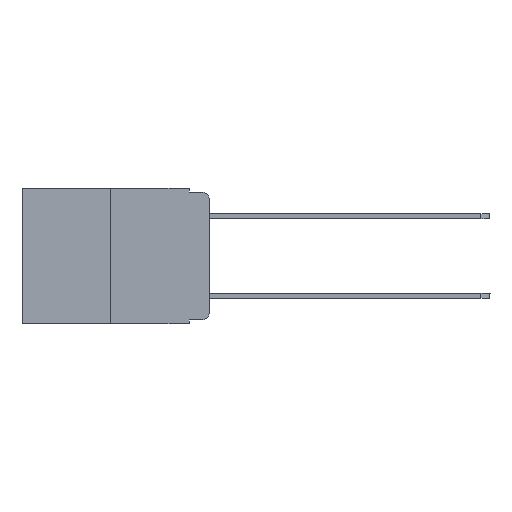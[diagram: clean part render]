
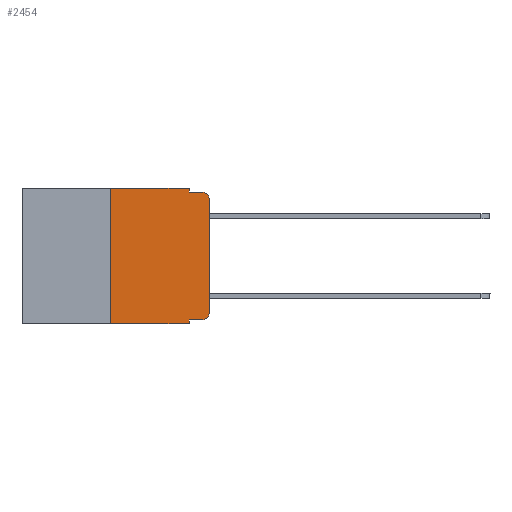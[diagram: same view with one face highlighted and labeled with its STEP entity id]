
A CAD part, left-side view. The second image highlights one B-rep face of the part: STEP entity #2454.
In plain terms, the highlighted planar face has unit normal (-1, 0, 0).
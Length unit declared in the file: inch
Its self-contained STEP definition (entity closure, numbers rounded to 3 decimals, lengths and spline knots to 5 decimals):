
#126 = VERTEX_POINT ( 'NONE', #4858 ) ;
#336 = ORIENTED_EDGE ( 'NONE', *, *, #6059, .T. ) ;
#388 = ORIENTED_EDGE ( 'NONE', *, *, #6709, .T. ) ;
#465 = EDGE_LOOP ( 'NONE', ( #6088, #12707, #9747, #11387, #4424, #7890, #388, #7771, #10635, #336 ) ) ;
#998 = CARTESIAN_POINT ( 'NONE',  ( 0., 0.02, -0.313 ) ) ;
#1402 = CARTESIAN_POINT ( 'NONE',  ( 0., 0.02, -0.01 ) ) ;
#1640 = EDGE_CURVE ( 'NONE', #2053, #11706, #2473, .T. ) ;
#1708 = AXIS2_PLACEMENT_3D ( 'NONE', #2082, #2881, #10051 ) ;
#1828 = CARTESIAN_POINT ( 'NONE',  ( 0., 0., 0. ) ) ;
#2053 = VERTEX_POINT ( 'NONE', #12426 ) ;
#2082 = CARTESIAN_POINT ( 'NONE',  ( 0., 0.473, 0. ) ) ;
#2126 = LINE ( 'NONE', #8281, #8659 ) ;
#2194 = DIRECTION ( 'NONE',  ( 0., 0., -1. ) ) ;
#2251 = DIRECTION ( 'NONE',  ( 0., -1., 0. ) ) ;
#2450 = CARTESIAN_POINT ( 'NONE',  ( 0., 0.02, -0.333 ) ) ;
#2454 = ADVANCED_FACE ( 'NONE', ( #8114 ), #12247, .F. ) ;
#2473 = CIRCLE ( 'NONE', #4181, 0.02 ) ;
#2568 = VERTEX_POINT ( 'NONE', #12329 ) ;
#2829 = EDGE_CURVE ( 'NONE', #126, #2053, #10996, .T. ) ;
#2830 = LINE ( 'NONE', #11875, #12501 ) ;
#2881 = DIRECTION ( 'NONE',  ( 1., 0., 0. ) ) ;
#2900 = DIRECTION ( 'NONE',  ( 0., -1., 0. ) ) ;
#3019 = EDGE_CURVE ( 'NONE', #10399, #3086, #12302, .T. ) ;
#3086 = VERTEX_POINT ( 'NONE', #3205 ) ;
#3125 = VECTOR ( 'NONE', #7096, 39.37008 ) ;
#3205 = CARTESIAN_POINT ( 'NONE',  ( 0., 0.25, 0. ) ) ;
#3327 = DIRECTION ( 'NONE',  ( -1., 0., 0. ) ) ;
#3738 = CARTESIAN_POINT ( 'NONE',  ( 0., 0.051, 0. ) ) ;
#3748 = CARTESIAN_POINT ( 'NONE',  ( 0., 0.051, 0. ) ) ;
#3861 = VERTEX_POINT ( 'NONE', #10927 ) ;
#3913 = VECTOR ( 'NONE', #8777, 39.37008 ) ;
#4181 = AXIS2_PLACEMENT_3D ( 'NONE', #9445, #3327, #2194 ) ;
#4343 = VERTEX_POINT ( 'NONE', #3748 ) ;
#4424 = ORIENTED_EDGE ( 'NONE', *, *, #11277, .F. ) ;
#4569 = CARTESIAN_POINT ( 'NONE',  ( 0., 0.051, -0.343 ) ) ;
#4829 = LINE ( 'NONE', #12912, #8222 ) ;
#4858 = CARTESIAN_POINT ( 'NONE',  ( 0., 0., -0.313 ) ) ;
#5090 = DIRECTION ( 'NONE',  ( -1., 0., 0. ) ) ;
#5369 = VERTEX_POINT ( 'NONE', #4569 ) ;
#5817 = EDGE_CURVE ( 'NONE', #4343, #2568, #9903, .T. ) ;
#5929 = EDGE_CURVE ( 'NONE', #3861, #5369, #9705, .T. ) ;
#6059 = EDGE_CURVE ( 'NONE', #7695, #126, #11404, .T. ) ;
#6088 = ORIENTED_EDGE ( 'NONE', *, *, #2829, .T. ) ;
#6276 = CARTESIAN_POINT ( 'NONE',  ( 0., 0.473, 0. ) ) ;
#6494 = CARTESIAN_POINT ( 'NONE',  ( 0., 0.25, -0.343 ) ) ;
#6709 = EDGE_CURVE ( 'NONE', #10399, #5369, #4829, .T. ) ;
#6982 = VECTOR ( 'NONE', #2251, 39.37008 ) ;
#7096 = DIRECTION ( 'NONE',  ( 0., 0., 1. ) ) ;
#7585 = EDGE_CURVE ( 'NONE', #2568, #11706, #2126, .T. ) ;
#7695 = VERTEX_POINT ( 'NONE', #2450 ) ;
#7738 = DIRECTION ( 'NONE',  ( 0., -1., 0. ) ) ;
#7771 = ORIENTED_EDGE ( 'NONE', *, *, #5929, .F. ) ;
#7775 = VECTOR ( 'NONE', #7841, 39.37008 ) ;
#7833 = EDGE_CURVE ( 'NONE', #3861, #7695, #2830, .T. ) ;
#7841 = DIRECTION ( 'NONE',  ( 0., 0., -1. ) ) ;
#7890 = ORIENTED_EDGE ( 'NONE', *, *, #3019, .F. ) ;
#8114 = FACE_OUTER_BOUND ( 'NONE', #465, .T. ) ;
#8222 = VECTOR ( 'NONE', #7738, 39.37008 ) ;
#8281 = CARTESIAN_POINT ( 'NONE',  ( 0., 0.051, -0.01 ) ) ;
#8659 = VECTOR ( 'NONE', #9230, 39.37008 ) ;
#8777 = DIRECTION ( 'NONE',  ( 0., 0., -1. ) ) ;
#8861 = DIRECTION ( 'NONE',  ( 0., 0., 1. ) ) ;
#9230 = DIRECTION ( 'NONE',  ( 0., -1., 0. ) ) ;
#9281 = AXIS2_PLACEMENT_3D ( 'NONE', #998, #5090, #13234 ) ;
#9445 = CARTESIAN_POINT ( 'NONE',  ( 0., 0.02, -0.03 ) ) ;
#9509 = VECTOR ( 'NONE', #8861, 39.37008 ) ;
#9705 = LINE ( 'NONE', #3738, #7775 ) ;
#9747 = ORIENTED_EDGE ( 'NONE', *, *, #7585, .F. ) ;
#9903 = LINE ( 'NONE', #12964, #3913 ) ;
#10051 = DIRECTION ( 'NONE',  ( 0., 0., -1. ) ) ;
#10399 = VERTEX_POINT ( 'NONE', #6494 ) ;
#10635 = ORIENTED_EDGE ( 'NONE', *, *, #7833, .T. ) ;
#10927 = CARTESIAN_POINT ( 'NONE',  ( 0., 0.051, -0.333 ) ) ;
#10996 = LINE ( 'NONE', #1828, #9509 ) ;
#11277 = EDGE_CURVE ( 'NONE', #3086, #4343, #13206, .T. ) ;
#11387 = ORIENTED_EDGE ( 'NONE', *, *, #5817, .F. ) ;
#11404 = CIRCLE ( 'NONE', #9281, 0.02 ) ;
#11706 = VERTEX_POINT ( 'NONE', #1402 ) ;
#11875 = CARTESIAN_POINT ( 'NONE',  ( 0., 0.051, -0.333 ) ) ;
#12247 = PLANE ( 'NONE',  #1708 ) ;
#12302 = LINE ( 'NONE', #13228, #3125 ) ;
#12329 = CARTESIAN_POINT ( 'NONE',  ( 0., 0.051, -0.01 ) ) ;
#12426 = CARTESIAN_POINT ( 'NONE',  ( 0., 0., -0.03 ) ) ;
#12501 = VECTOR ( 'NONE', #2900, 39.37008 ) ;
#12707 = ORIENTED_EDGE ( 'NONE', *, *, #1640, .T. ) ;
#12912 = CARTESIAN_POINT ( 'NONE',  ( 0., 0.473, -0.343 ) ) ;
#12964 = CARTESIAN_POINT ( 'NONE',  ( 0., 0.051, 0. ) ) ;
#13206 = LINE ( 'NONE', #6276, #6982 ) ;
#13228 = CARTESIAN_POINT ( 'NONE',  ( 0., 0.25, 0. ) ) ;
#13234 = DIRECTION ( 'NONE',  ( 0., 0., -1. ) ) ;
